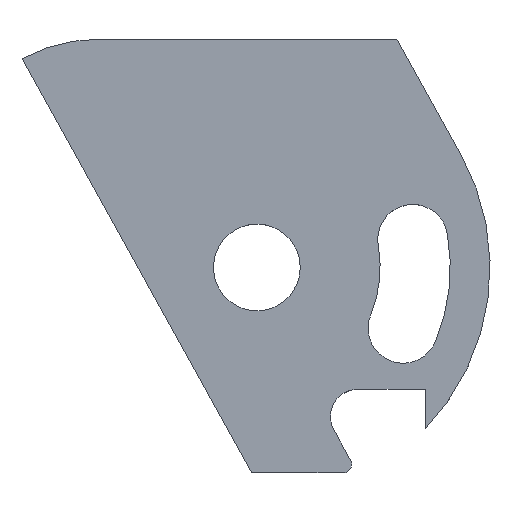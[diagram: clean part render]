
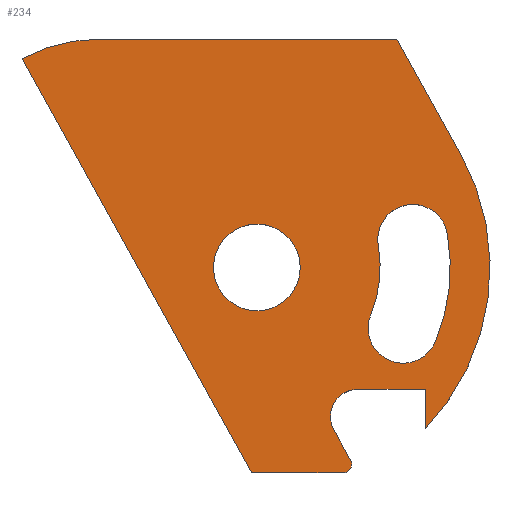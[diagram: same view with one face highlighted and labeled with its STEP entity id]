
A CAD part, top view. The second image highlights one B-rep face of the part: STEP entity #234.
In plain terms, the highlighted planar face has unit normal (0, 0, 1).
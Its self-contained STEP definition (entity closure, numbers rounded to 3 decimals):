
#2 = CIRCLE ( 'NONE', #177, 2.019 ) ;
#4 = ORIENTED_EDGE ( 'NONE', *, *, #441, .T. ) ;
#5 = ORIENTED_EDGE ( 'NONE', *, *, #421, .T. ) ;
#16 = ORIENTED_EDGE ( 'NONE', *, *, #399, .T. ) ;
#19 = DIRECTION ( 'NONE',  ( 1., 0., 0. ) ) ;
#22 = VERTEX_POINT ( 'NONE', #288 ) ;
#27 = ORIENTED_EDGE ( 'NONE', *, *, #488, .T. ) ;
#34 = ORIENTED_EDGE ( 'NONE', *, *, #504, .T. ) ;
#36 = LINE ( 'NONE', #586, #439 ) ;
#37 = CARTESIAN_POINT ( 'NONE',  ( -0.246, -9.563, 0.654 ) ) ;
#39 = VERTEX_POINT ( 'NONE', #218 ) ;
#45 = CARTESIAN_POINT ( 'NONE',  ( -7.32, 10.63, 0.654 ) ) ;
#50 = VERTEX_POINT ( 'NONE', #351 ) ;
#52 = DIRECTION ( 'NONE',  ( 0., -1., 0. ) ) ;
#57 = ORIENTED_EDGE ( 'NONE', *, *, #503, .T. ) ;
#59 = ORIENTED_EDGE ( 'NONE', *, *, #419, .T. ) ;
#65 = DIRECTION ( 'NONE',  ( 0.923, -0.384, 0. ) ) ;
#68 = CARTESIAN_POINT ( 'NONE',  ( 7.847, -7.506, 0.654 ) ) ;
#77 = ORIENTED_EDGE ( 'NONE', *, *, #407, .T. ) ;
#82 = DIRECTION ( 'NONE',  ( 0.485, -0.875, 0. ) ) ;
#90 = VERTEX_POINT ( 'NONE', #278 ) ;
#94 = CARTESIAN_POINT ( 'NONE',  ( -2.019, 0., 0.654 ) ) ;
#97 = VECTOR ( 'NONE', #611, 1000. ) ;
#98 = DIRECTION ( 'NONE',  ( 0., -1., 0. ) ) ;
#100 = ORIENTED_EDGE ( 'NONE', *, *, #403, .T. ) ;
#104 = FACE_BOUND ( 'NONE', #316, .T. ) ;
#107 = CARTESIAN_POINT ( 'NONE',  ( 7.847, -7.506, 0.654 ) ) ;
#114 = CARTESIAN_POINT ( 'NONE',  ( 0., 0., 0.654 ) ) ;
#121 = VERTEX_POINT ( 'NONE', #355 ) ;
#128 = VERTEX_POINT ( 'NONE', #361 ) ;
#134 = CIRCLE ( 'NONE', #154, 5.74 ) ;
#136 = CARTESIAN_POINT ( 'NONE',  ( 4.017, -9.166, 0.654 ) ) ;
#138 = CIRCLE ( 'NONE', #192, 2.019 ) ;
#139 = CARTESIAN_POINT ( 'NONE',  ( 0., 0., 0.654 ) ) ;
#143 = DIRECTION ( 'NONE',  ( 0., 0., 1. ) ) ;
#146 = CARTESIAN_POINT ( 'NONE',  ( -0.246, -9.563, 0.654 ) ) ;
#147 = VERTEX_POINT ( 'NONE', #107 ) ;
#152 = ORIENTED_EDGE ( 'NONE', *, *, #392, .T. ) ;
#154 = AXIS2_PLACEMENT_3D ( 'NONE', #424, #422, #420 ) ;
#155 = CARTESIAN_POINT ( 'NONE',  ( 6.523, 10.63, 0.654 ) ) ;
#156 = AXIS2_PLACEMENT_3D ( 'NONE', #447, #442, #437 ) ;
#158 = AXIS2_PLACEMENT_3D ( 'NONE', #508, #507, #506 ) ;
#165 = VERTEX_POINT ( 'NONE', #658 ) ;
#168 = AXIS2_PLACEMENT_3D ( 'NONE', #630, #626, #624 ) ;
#170 = AXIS2_PLACEMENT_3D ( 'NONE', #114, #543, #65 ) ;
#173 = DIRECTION ( 'NONE',  ( -1., 0., 0. ) ) ;
#174 = AXIS2_PLACEMENT_3D ( 'NONE', #416, #143, #98 ) ;
#177 = AXIS2_PLACEMENT_3D ( 'NONE', #139, #551, #578 ) ;
#184 = AXIS2_PLACEMENT_3D ( 'NONE', #136, #513, #381 ) ;
#190 = AXIS2_PLACEMENT_3D ( 'NONE', #559, #645, #566 ) ;
#192 = AXIS2_PLACEMENT_3D ( 'NONE', #571, #259, #173 ) ;
#204 = CIRCLE ( 'NONE', #168, 10.858 ) ;
#216 = LINE ( 'NONE', #146, #380 ) ;
#218 = CARTESIAN_POINT ( 'NONE',  ( 3.582, -7.563, 0.654 ) ) ;
#234 = ADVANCED_FACE ( 'NONE', ( #579, #104, #252 ), #313, .T. ) ;
#235 = CIRCLE ( 'NONE', #170, 9.004 ) ;
#252 = FACE_BOUND ( 'NONE', #274, .T. ) ;
#259 = DIRECTION ( 'NONE',  ( 0., 0., -1. ) ) ;
#261 = CARTESIAN_POINT ( 'NONE',  ( 0.833, 1.615, 0.654 ) ) ;
#265 = VERTEX_POINT ( 'NONE', #371 ) ;
#274 = EDGE_LOOP ( 'NONE', ( #16, #326 ) ) ;
#278 = CARTESIAN_POINT ( 'NONE',  ( 4.017, -9.563, 0.654 ) ) ;
#279 = VERTEX_POINT ( 'NONE', #94 ) ;
#288 = CARTESIAN_POINT ( 'NONE',  ( -10.935, 9.72, 0.654 ) ) ;
#295 = ORIENTED_EDGE ( 'NONE', *, *, #471, .T. ) ;
#299 = EDGE_LOOP ( 'NONE', ( #295, #432, #470, #491, #577, #5, #59, #77, #100, #152, #329 ) ) ;
#300 = VECTOR ( 'NONE', #463, 1000. ) ;
#313 = PLANE ( 'NONE',  #315 ) ;
#315 = AXIS2_PLACEMENT_3D ( 'NONE', #261, #524, #614 ) ;
#316 = EDGE_LOOP ( 'NONE', ( #57, #34, #27, #4 ) ) ;
#322 = VERTEX_POINT ( 'NONE', #580 ) ;
#326 = ORIENTED_EDGE ( 'NONE', *, *, #429, .T. ) ;
#329 = ORIENTED_EDGE ( 'NONE', *, *, #385, .T. ) ;
#331 = CIRCLE ( 'NONE', #156, 1.632 ) ;
#334 = LINE ( 'NONE', #68, #607 ) ;
#345 = CARTESIAN_POINT ( 'NONE',  ( 6.523, 10.63, 0.654 ) ) ;
#351 = CARTESIAN_POINT ( 'NONE',  ( 4.364, -8.974, 0.654 ) ) ;
#355 = CARTESIAN_POINT ( 'NONE',  ( 8.315, -3.454, 0.654 ) ) ;
#356 = VERTEX_POINT ( 'NONE', #37 ) ;
#361 = CARTESIAN_POINT ( 'NONE',  ( 5.651, 1.012, 0.654 ) ) ;
#371 = CARTESIAN_POINT ( 'NONE',  ( 9.497, 5.264, 0.654 ) ) ;
#376 = VERTEX_POINT ( 'NONE', #155 ) ;
#380 = VECTOR ( 'NONE', #82, 1000. ) ;
#381 = DIRECTION ( 'NONE',  ( 0., 1., 0. ) ) ;
#385 = EDGE_CURVE ( 'NONE', #498, #147, #334, .T. ) ;
#392 = EDGE_CURVE ( 'NONE', #165, #498, #479, .T. ) ;
#399 = EDGE_CURVE ( 'NONE', #279, #485, #138, .T. ) ;
#400 = VERTEX_POINT ( 'NONE', #45 ) ;
#403 = EDGE_CURVE ( 'NONE', #39, #165, #593, .T. ) ;
#407 = EDGE_CURVE ( 'NONE', #50, #39, #36, .T. ) ;
#411 = CARTESIAN_POINT ( 'NONE',  ( 5.301, -2.202, 0.654 ) ) ;
#416 = CARTESIAN_POINT ( 'NONE',  ( -7.32, 2.997, 0.654 ) ) ;
#419 = EDGE_CURVE ( 'NONE', #90, #50, #581, .T. ) ;
#420 = DIRECTION ( 'NONE',  ( -0.923, 0.384, 0. ) ) ;
#421 = EDGE_CURVE ( 'NONE', #356, #90, #423, .T. ) ;
#422 = DIRECTION ( 'NONE',  ( 0., 0., 1. ) ) ;
#423 = LINE ( 'NONE', #472, #97 ) ;
#424 = CARTESIAN_POINT ( 'NONE',  ( 0., 0., 0.654 ) ) ;
#429 = EDGE_CURVE ( 'NONE', #485, #279, #2, .T. ) ;
#431 = EDGE_CURVE ( 'NONE', #400, #22, #557, .T. ) ;
#432 = ORIENTED_EDGE ( 'NONE', *, *, #467, .T. ) ;
#437 = DIRECTION ( 'NONE',  ( -0.923, 0.384, 0. ) ) ;
#439 = VECTOR ( 'NONE', #620, 1000. ) ;
#441 = EDGE_CURVE ( 'NONE', #322, #121, #235, .T. ) ;
#442 = DIRECTION ( 'NONE',  ( 0., 0., -1. ) ) ;
#447 = CARTESIAN_POINT ( 'NONE',  ( 6.808, -2.828, 0.654 ) ) ;
#448 = EDGE_CURVE ( 'NONE', #22, #356, #216, .T. ) ;
#463 = DIRECTION ( 'NONE',  ( -1., 0., 0. ) ) ;
#467 = EDGE_CURVE ( 'NONE', #265, #376, #643, .T. ) ;
#470 = ORIENTED_EDGE ( 'NONE', *, *, #499, .T. ) ;
#471 = EDGE_CURVE ( 'NONE', #147, #265, #204, .T. ) ;
#472 = CARTESIAN_POINT ( 'NONE',  ( 4.017, -9.563, 0.654 ) ) ;
#477 = LINE ( 'NONE', #546, #300 ) ;
#479 = LINE ( 'NONE', #512, #501 ) ;
#485 = VERTEX_POINT ( 'NONE', #575 ) ;
#488 = EDGE_CURVE ( 'NONE', #128, #322, #500, .T. ) ;
#491 = ORIENTED_EDGE ( 'NONE', *, *, #431, .T. ) ;
#494 = CARTESIAN_POINT ( 'NONE',  ( 7.847, -5.677, 0.654 ) ) ;
#498 = VERTEX_POINT ( 'NONE', #494 ) ;
#499 = EDGE_CURVE ( 'NONE', #376, #400, #477, .T. ) ;
#500 = CIRCLE ( 'NONE', #158, 1.632 ) ;
#501 = VECTOR ( 'NONE', #19, 1000. ) ;
#503 = EDGE_CURVE ( 'NONE', #121, #535, #331, .T. ) ;
#504 = EDGE_CURVE ( 'NONE', #535, #128, #134, .T. ) ;
#506 = DIRECTION ( 'NONE',  ( 0.984, 0.176, 0. ) ) ;
#507 = DIRECTION ( 'NONE',  ( 0., 0., -1. ) ) ;
#508 = CARTESIAN_POINT ( 'NONE',  ( 7.257, 1.299, 0.654 ) ) ;
#512 = CARTESIAN_POINT ( 'NONE',  ( 7.847, -5.677, 0.654 ) ) ;
#513 = DIRECTION ( 'NONE',  ( 0., 0., 1. ) ) ;
#524 = DIRECTION ( 'NONE',  ( 0., 0., 1. ) ) ;
#531 = VECTOR ( 'NONE', #534, 1000. ) ;
#534 = DIRECTION ( 'NONE',  ( -0.485, 0.875, 0. ) ) ;
#535 = VERTEX_POINT ( 'NONE', #411 ) ;
#543 = DIRECTION ( 'NONE',  ( 0., 0., -1. ) ) ;
#546 = CARTESIAN_POINT ( 'NONE',  ( -7.32, 10.63, 0.654 ) ) ;
#551 = DIRECTION ( 'NONE',  ( 0., 0., -1. ) ) ;
#557 = CIRCLE ( 'NONE', #174, 7.633 ) ;
#559 = CARTESIAN_POINT ( 'NONE',  ( 4.693, -6.947, 0.654 ) ) ;
#566 = DIRECTION ( 'NONE',  ( 0., 1., 0. ) ) ;
#571 = CARTESIAN_POINT ( 'NONE',  ( 0., 0., 0.654 ) ) ;
#575 = CARTESIAN_POINT ( 'NONE',  ( 2.019, 0., 0.654 ) ) ;
#577 = ORIENTED_EDGE ( 'NONE', *, *, #448, .T. ) ;
#578 = DIRECTION ( 'NONE',  ( -1., 0., 0. ) ) ;
#579 = FACE_OUTER_BOUND ( 'NONE', #299, .T. ) ;
#580 = CARTESIAN_POINT ( 'NONE',  ( 8.863, 1.587, 0.654 ) ) ;
#581 = CIRCLE ( 'NONE', #184, 0.397 ) ;
#586 = CARTESIAN_POINT ( 'NONE',  ( 3.582, -7.563, 0.654 ) ) ;
#593 = CIRCLE ( 'NONE', #190, 1.27 ) ;
#607 = VECTOR ( 'NONE', #52, 1000. ) ;
#611 = DIRECTION ( 'NONE',  ( 1., 0., 0. ) ) ;
#614 = DIRECTION ( 'NONE',  ( 1., 0., 0. ) ) ;
#620 = DIRECTION ( 'NONE',  ( -0.485, 0.875, 0. ) ) ;
#624 = DIRECTION ( 'NONE',  ( -0.723, 0.691, 0. ) ) ;
#626 = DIRECTION ( 'NONE',  ( 0., 0., 1. ) ) ;
#630 = CARTESIAN_POINT ( 'NONE',  ( 0., 0., 0.654 ) ) ;
#643 = LINE ( 'NONE', #345, #531 ) ;
#645 = DIRECTION ( 'NONE',  ( 0., 0., -1. ) ) ;
#658 = CARTESIAN_POINT ( 'NONE',  ( 4.693, -5.677, 0.654 ) ) ;
